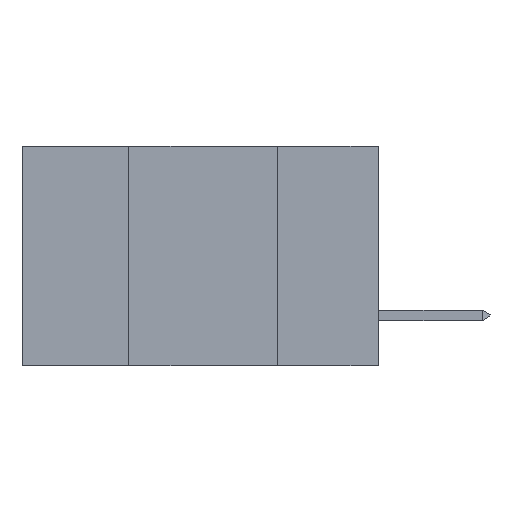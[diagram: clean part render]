
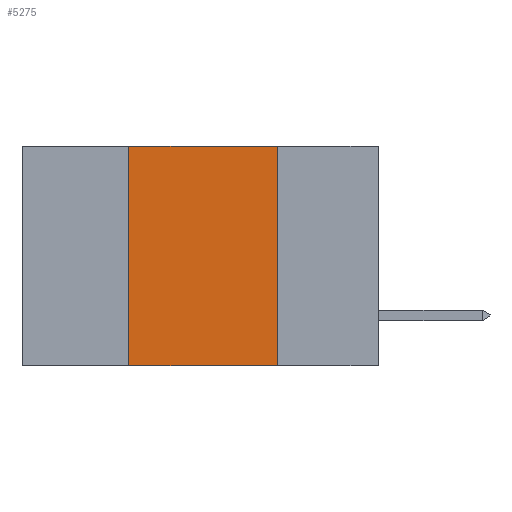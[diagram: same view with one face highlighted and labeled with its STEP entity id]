
A CAD part, left-side view. The second image highlights one B-rep face of the part: STEP entity #5275.
In plain terms, the highlighted planar face has unit normal (-1, 0, 0).
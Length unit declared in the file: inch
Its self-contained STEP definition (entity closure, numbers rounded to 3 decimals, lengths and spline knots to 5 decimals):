
#209 = LINE ( 'NONE', #10038, #10216 ) ;
#500 = CARTESIAN_POINT ( 'NONE',  ( 0., 0.17, -0.37 ) ) ;
#1013 = ORIENTED_EDGE ( 'NONE', *, *, #3569, .F. ) ;
#1507 = CARTESIAN_POINT ( 'NONE',  ( 0., 0.42, -0.37 ) ) ;
#1555 = DIRECTION ( 'NONE',  ( 0., 0., -1. ) ) ;
#3569 = EDGE_CURVE ( 'NONE', #7696, #16006, #16120, .T. ) ;
#4188 = DIRECTION ( 'NONE',  ( 0., 0., 1. ) ) ;
#4318 = DIRECTION ( 'NONE',  ( 1., 0., 0. ) ) ;
#4814 = VERTEX_POINT ( 'NONE', #4836 ) ;
#4836 = CARTESIAN_POINT ( 'NONE',  ( 0., 0.42, -0.37 ) ) ;
#5002 = ORIENTED_EDGE ( 'NONE', *, *, #5050, .T. ) ;
#5050 = EDGE_CURVE ( 'NONE', #4814, #10648, #209, .T. ) ;
#5275 = ADVANCED_FACE ( 'NONE', ( #6997 ), #5791, .F. ) ;
#5338 = ORIENTED_EDGE ( 'NONE', *, *, #11421, .F. ) ;
#5791 = PLANE ( 'NONE',  #18218 ) ;
#6827 = DIRECTION ( 'NONE',  ( 0., -1., 0. ) ) ;
#6997 = FACE_OUTER_BOUND ( 'NONE', #14510, .T. ) ;
#7696 = VERTEX_POINT ( 'NONE', #15741 ) ;
#8249 = ORIENTED_EDGE ( 'NONE', *, *, #10509, .F. ) ;
#8742 = DIRECTION ( 'NONE',  ( 0., -1., 0. ) ) ;
#10031 = LINE ( 'NONE', #17191, #10415 ) ;
#10038 = CARTESIAN_POINT ( 'NONE',  ( 0., 0.6, -0.37 ) ) ;
#10216 = VECTOR ( 'NONE', #8742, 39.37008 ) ;
#10415 = VECTOR ( 'NONE', #1555, 39.37008 ) ;
#10509 = EDGE_CURVE ( 'NONE', #4814, #7696, #11329, .T. ) ;
#10648 = VERTEX_POINT ( 'NONE', #500 ) ;
#11187 = DIRECTION ( 'NONE',  ( 0., 0., -1. ) ) ;
#11259 = VECTOR ( 'NONE', #6827, 39.37008 ) ;
#11329 = LINE ( 'NONE', #1507, #13687 ) ;
#11421 = EDGE_CURVE ( 'NONE', #16006, #10648, #10031, .T. ) ;
#13687 = VECTOR ( 'NONE', #4188, 39.37008 ) ;
#14510 = EDGE_LOOP ( 'NONE', ( #5338, #1013, #8249, #5002 ) ) ;
#14725 = CARTESIAN_POINT ( 'NONE',  ( 0., 0.6, 0. ) ) ;
#15741 = CARTESIAN_POINT ( 'NONE',  ( 0., 0.42, 0. ) ) ;
#16006 = VERTEX_POINT ( 'NONE', #16222 ) ;
#16120 = LINE ( 'NONE', #14725, #11259 ) ;
#16222 = CARTESIAN_POINT ( 'NONE',  ( 0., 0.17, 0. ) ) ;
#17025 = CARTESIAN_POINT ( 'NONE',  ( 0., 0.6, 0. ) ) ;
#17191 = CARTESIAN_POINT ( 'NONE',  ( 0., 0.17, -0.37 ) ) ;
#18218 = AXIS2_PLACEMENT_3D ( 'NONE', #17025, #4318, #11187 ) ;
